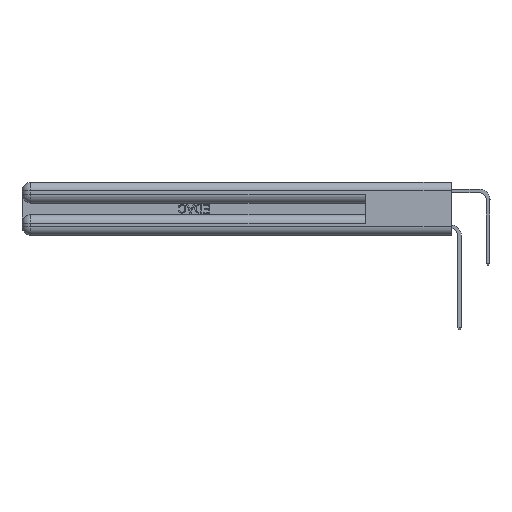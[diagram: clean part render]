
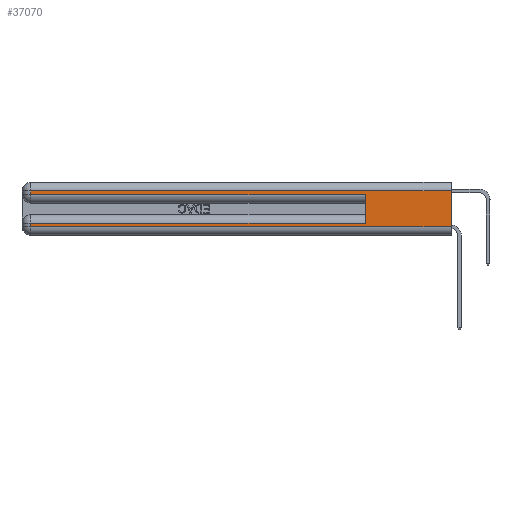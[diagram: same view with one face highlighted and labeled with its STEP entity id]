
A CAD part, left-side view. The second image highlights one B-rep face of the part: STEP entity #37070.
In plain terms, the highlighted planar face has unit normal (-1, 0, 0).
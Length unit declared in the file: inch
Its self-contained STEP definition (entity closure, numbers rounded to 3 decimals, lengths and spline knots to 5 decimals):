
#173 = LINE ( 'NONE', #24709, #30925 ) ;
#254 = DIRECTION ( 'NONE',  ( 0., -1., 0. ) ) ;
#916 = LINE ( 'NONE', #25331, #1403 ) ;
#1320 = VERTEX_POINT ( 'NONE', #30281 ) ;
#1403 = VECTOR ( 'NONE', #1535, 39.37008 ) ;
#1535 = DIRECTION ( 'NONE',  ( 0., 1., 0. ) ) ;
#2832 = DIRECTION ( 'NONE',  ( 0., 0., -1. ) ) ;
#3509 = DIRECTION ( 'NONE',  ( 0., 0., -1. ) ) ;
#3562 = EDGE_CURVE ( 'NONE', #36270, #9736, #31691, .T. ) ;
#5173 = AXIS2_PLACEMENT_3D ( 'NONE', #35238, #35309, #14901 ) ;
#5529 = DIRECTION ( 'NONE',  ( 0., 0., 1. ) ) ;
#5851 = VECTOR ( 'NONE', #2832, 39.37008 ) ;
#5908 = ORIENTED_EDGE ( 'NONE', *, *, #23868, .T. ) ;
#6177 = VECTOR ( 'NONE', #254, 39.37008 ) ;
#9736 = VERTEX_POINT ( 'NONE', #10826 ) ;
#10777 = CARTESIAN_POINT ( 'NONE',  ( 0., 2.94, 0.085 ) ) ;
#10826 = CARTESIAN_POINT ( 'NONE',  ( 0., 0., 0.06 ) ) ;
#11628 = VERTEX_POINT ( 'NONE', #27203 ) ;
#12195 = EDGE_LOOP ( 'NONE', ( #33074, #18994, #5908, #24952, #18301, #38169, #17834, #22832 ) ) ;
#14901 = DIRECTION ( 'NONE',  ( 0., 0., -1. ) ) ;
#15263 = DIRECTION ( 'NONE',  ( 0., 0., -1. ) ) ;
#15501 = FACE_OUTER_BOUND ( 'NONE', #12195, .T. ) ;
#16324 = VECTOR ( 'NONE', #37487, 39.37008 ) ;
#16782 = CARTESIAN_POINT ( 'NONE',  ( 0., 0., 0.31 ) ) ;
#17042 = CARTESIAN_POINT ( 'NONE',  ( 0., 2.94, 0.31 ) ) ;
#17834 = ORIENTED_EDGE ( 'NONE', *, *, #36356, .T. ) ;
#18301 = ORIENTED_EDGE ( 'NONE', *, *, #25367, .F. ) ;
#18833 = VECTOR ( 'NONE', #5529, 39.37008 ) ;
#18994 = ORIENTED_EDGE ( 'NONE', *, *, #19602, .T. ) ;
#19537 = VECTOR ( 'NONE', #15263, 39.37008 ) ;
#19602 = EDGE_CURVE ( 'NONE', #36270, #35620, #21403, .T. ) ;
#19812 = CARTESIAN_POINT ( 'NONE',  ( 0., 0.6, 0.285 ) ) ;
#20664 = LINE ( 'NONE', #35611, #5851 ) ;
#20685 = VERTEX_POINT ( 'NONE', #10777 ) ;
#21403 = LINE ( 'NONE', #16782, #16324 ) ;
#21567 = DIRECTION ( 'NONE',  ( 0., -1., 0. ) ) ;
#22832 = ORIENTED_EDGE ( 'NONE', *, *, #29075, .T. ) ;
#23301 = CARTESIAN_POINT ( 'NONE',  ( 0., 0.6, 0.145 ) ) ;
#23868 = EDGE_CURVE ( 'NONE', #35620, #35968, #36121, .T. ) ;
#24709 = CARTESIAN_POINT ( 'NONE',  ( 0., 0., 0.285 ) ) ;
#24952 = ORIENTED_EDGE ( 'NONE', *, *, #26133, .T. ) ;
#25331 = CARTESIAN_POINT ( 'NONE',  ( 0., 0., 0.085 ) ) ;
#25367 = EDGE_CURVE ( 'NONE', #11628, #31646, #26764, .T. ) ;
#26133 = EDGE_CURVE ( 'NONE', #35968, #31646, #173, .T. ) ;
#26764 = LINE ( 'NONE', #23301, #18833 ) ;
#27068 = CARTESIAN_POINT ( 'NONE',  ( 0., 0., 0.37 ) ) ;
#27203 = CARTESIAN_POINT ( 'NONE',  ( 0., 0.6, 0.085 ) ) ;
#29075 = EDGE_CURVE ( 'NONE', #1320, #9736, #29906, .T. ) ;
#29160 = VECTOR ( 'NONE', #3509, 39.37008 ) ;
#29906 = LINE ( 'NONE', #35680, #6177 ) ;
#30060 = CARTESIAN_POINT ( 'NONE',  ( 0., 2.94, 0.37 ) ) ;
#30281 = CARTESIAN_POINT ( 'NONE',  ( 0., 2.94, 0.06 ) ) ;
#30875 = EDGE_CURVE ( 'NONE', #11628, #20685, #916, .T. ) ;
#30925 = VECTOR ( 'NONE', #21567, 39.37008 ) ;
#31646 = VERTEX_POINT ( 'NONE', #19812 ) ;
#31691 = LINE ( 'NONE', #27068, #19537 ) ;
#32224 = CARTESIAN_POINT ( 'NONE',  ( 0., 0., 0.31 ) ) ;
#32707 = PLANE ( 'NONE',  #5173 ) ;
#33074 = ORIENTED_EDGE ( 'NONE', *, *, #3562, .F. ) ;
#33421 = CARTESIAN_POINT ( 'NONE',  ( 0., 2.94, 0.285 ) ) ;
#35238 = CARTESIAN_POINT ( 'NONE',  ( 0., 0., 0.37 ) ) ;
#35309 = DIRECTION ( 'NONE',  ( 1., 0., 0. ) ) ;
#35611 = CARTESIAN_POINT ( 'NONE',  ( 0., 2.94, 0.37 ) ) ;
#35620 = VERTEX_POINT ( 'NONE', #17042 ) ;
#35680 = CARTESIAN_POINT ( 'NONE',  ( 0., 0., 0.06 ) ) ;
#35968 = VERTEX_POINT ( 'NONE', #33421 ) ;
#36121 = LINE ( 'NONE', #30060, #29160 ) ;
#36270 = VERTEX_POINT ( 'NONE', #32224 ) ;
#36356 = EDGE_CURVE ( 'NONE', #20685, #1320, #20664, .T. ) ;
#37070 = ADVANCED_FACE ( 'NONE', ( #15501 ), #32707, .F. ) ;
#37487 = DIRECTION ( 'NONE',  ( 0., 1., 0. ) ) ;
#38169 = ORIENTED_EDGE ( 'NONE', *, *, #30875, .T. ) ;
